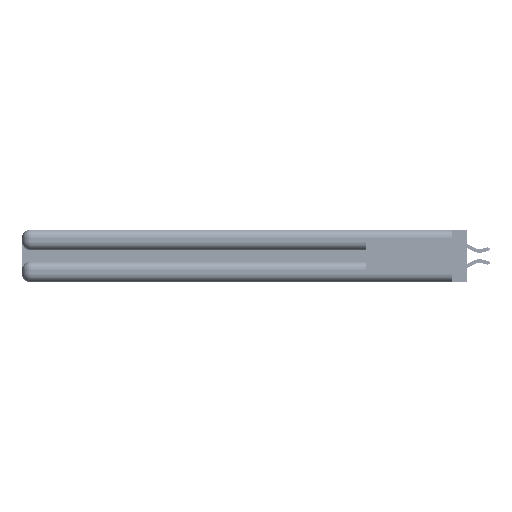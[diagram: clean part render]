
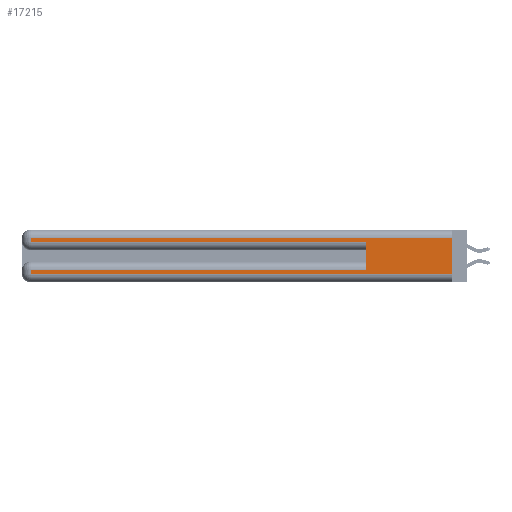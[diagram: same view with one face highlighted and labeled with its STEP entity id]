
A CAD part, left-side view. The second image highlights one B-rep face of the part: STEP entity #17215.
In plain terms, the highlighted planar face has unit normal (-1, 0, 0).
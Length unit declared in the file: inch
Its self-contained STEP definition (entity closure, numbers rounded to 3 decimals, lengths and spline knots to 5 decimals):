
#542 = CARTESIAN_POINT ( 'NONE',  ( 0., 0., 0.06 ) ) ;
#579 = LINE ( 'NONE', #45675, #24502 ) ;
#1467 = DIRECTION ( 'NONE',  ( 0., 0., -1. ) ) ;
#2036 = LINE ( 'NONE', #45290, #51804 ) ;
#2697 = DIRECTION ( 'NONE',  ( 0., 0., -1. ) ) ;
#3365 = EDGE_CURVE ( 'NONE', #28711, #39993, #21000, .T. ) ;
#4002 = EDGE_CURVE ( 'NONE', #28711, #15115, #22827, .T. ) ;
#4236 = CARTESIAN_POINT ( 'NONE',  ( 0., 0., 0.31 ) ) ;
#5687 = CARTESIAN_POINT ( 'NONE',  ( 0., 0.6, 0.085 ) ) ;
#6305 = ORIENTED_EDGE ( 'NONE', *, *, #33619, .T. ) ;
#7070 = EDGE_CURVE ( 'NONE', #33870, #39993, #579, .T. ) ;
#7584 = VERTEX_POINT ( 'NONE', #41223 ) ;
#7816 = LINE ( 'NONE', #28096, #29872 ) ;
#8407 = DIRECTION ( 'NONE',  ( 0., 0., -1. ) ) ;
#8957 = ORIENTED_EDGE ( 'NONE', *, *, #43335, .T. ) ;
#9900 = EDGE_CURVE ( 'NONE', #14827, #7584, #7816, .T. ) ;
#12259 = DIRECTION ( 'NONE',  ( 0., 0., 1. ) ) ;
#13773 = CARTESIAN_POINT ( 'NONE',  ( 0., 2.94, 0.37 ) ) ;
#14492 = CARTESIAN_POINT ( 'NONE',  ( 0., 0.6, 0.285 ) ) ;
#14827 = VERTEX_POINT ( 'NONE', #4236 ) ;
#15115 = VERTEX_POINT ( 'NONE', #17909 ) ;
#15241 = VECTOR ( 'NONE', #43503, 39.37008 ) ;
#17215 = ADVANCED_FACE ( 'NONE', ( #32894 ), #42638, .F. ) ;
#17909 = CARTESIAN_POINT ( 'NONE',  ( 0., 2.94, 0.085 ) ) ;
#19731 = VECTOR ( 'NONE', #12259, 39.37008 ) ;
#21000 = LINE ( 'NONE', #48001, #19731 ) ;
#21458 = ORIENTED_EDGE ( 'NONE', *, *, #7070, .T. ) ;
#22634 = EDGE_CURVE ( 'NONE', #15115, #23603, #2036, .T. ) ;
#22827 = LINE ( 'NONE', #27677, #15241 ) ;
#23102 = CARTESIAN_POINT ( 'NONE',  ( 0., 0., 0.37 ) ) ;
#23603 = VERTEX_POINT ( 'NONE', #30271 ) ;
#24060 = VECTOR ( 'NONE', #28690, 39.37008 ) ;
#24502 = VECTOR ( 'NONE', #37563, 39.37008 ) ;
#25781 = ORIENTED_EDGE ( 'NONE', *, *, #9900, .F. ) ;
#26779 = VECTOR ( 'NONE', #1467, 39.37008 ) ;
#27677 = CARTESIAN_POINT ( 'NONE',  ( 0., 0., 0.085 ) ) ;
#27761 = ORIENTED_EDGE ( 'NONE', *, *, #22634, .T. ) ;
#28035 = LINE ( 'NONE', #13773, #26779 ) ;
#28096 = CARTESIAN_POINT ( 'NONE',  ( 0., 0., 0.37 ) ) ;
#28264 = AXIS2_PLACEMENT_3D ( 'NONE', #23102, #38760, #2697 ) ;
#28689 = EDGE_CURVE ( 'NONE', #45831, #33870, #28035, .T. ) ;
#28690 = DIRECTION ( 'NONE',  ( 0., -1., 0. ) ) ;
#28711 = VERTEX_POINT ( 'NONE', #5687 ) ;
#29190 = CARTESIAN_POINT ( 'NONE',  ( 0., 0., 0.31 ) ) ;
#29872 = VECTOR ( 'NONE', #8407, 39.37008 ) ;
#30271 = CARTESIAN_POINT ( 'NONE',  ( 0., 2.94, 0.06 ) ) ;
#31910 = ORIENTED_EDGE ( 'NONE', *, *, #3365, .F. ) ;
#32894 = FACE_OUTER_BOUND ( 'NONE', #43858, .T. ) ;
#33619 = EDGE_CURVE ( 'NONE', #23603, #7584, #49909, .T. ) ;
#33870 = VERTEX_POINT ( 'NONE', #33959 ) ;
#33928 = ORIENTED_EDGE ( 'NONE', *, *, #4002, .T. ) ;
#33959 = CARTESIAN_POINT ( 'NONE',  ( 0., 2.94, 0.285 ) ) ;
#34591 = LINE ( 'NONE', #29190, #45892 ) ;
#37363 = DIRECTION ( 'NONE',  ( 0., 0., -1. ) ) ;
#37563 = DIRECTION ( 'NONE',  ( 0., -1., 0. ) ) ;
#38760 = DIRECTION ( 'NONE',  ( 1., 0., 0. ) ) ;
#39993 = VERTEX_POINT ( 'NONE', #14492 ) ;
#41162 = DIRECTION ( 'NONE',  ( 0., 1., 0. ) ) ;
#41223 = CARTESIAN_POINT ( 'NONE',  ( 0., 0., 0.06 ) ) ;
#42638 = PLANE ( 'NONE',  #28264 ) ;
#43335 = EDGE_CURVE ( 'NONE', #14827, #45831, #34591, .T. ) ;
#43503 = DIRECTION ( 'NONE',  ( 0., 1., 0. ) ) ;
#43858 = EDGE_LOOP ( 'NONE', ( #25781, #8957, #45035, #21458, #31910, #33928, #27761, #6305 ) ) ;
#45035 = ORIENTED_EDGE ( 'NONE', *, *, #28689, .T. ) ;
#45290 = CARTESIAN_POINT ( 'NONE',  ( 0., 2.94, 0.37 ) ) ;
#45675 = CARTESIAN_POINT ( 'NONE',  ( 0., 0., 0.285 ) ) ;
#45831 = VERTEX_POINT ( 'NONE', #47085 ) ;
#45892 = VECTOR ( 'NONE', #41162, 39.37008 ) ;
#47085 = CARTESIAN_POINT ( 'NONE',  ( 0., 2.94, 0.31 ) ) ;
#48001 = CARTESIAN_POINT ( 'NONE',  ( 0., 0.6, 0.145 ) ) ;
#49909 = LINE ( 'NONE', #542, #24060 ) ;
#51804 = VECTOR ( 'NONE', #37363, 39.37008 ) ;
